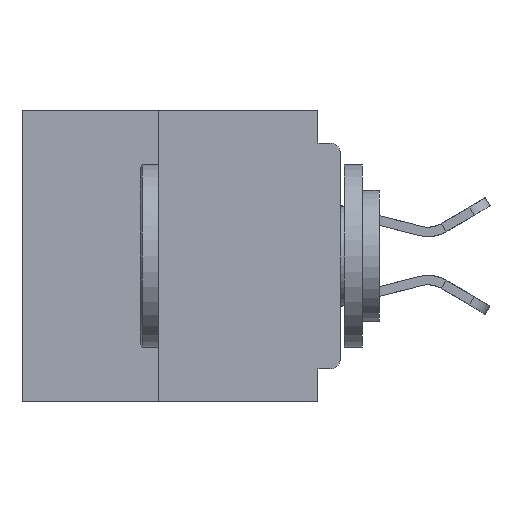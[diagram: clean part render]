
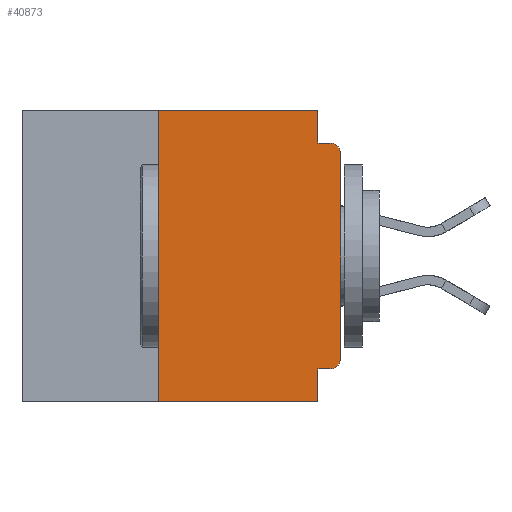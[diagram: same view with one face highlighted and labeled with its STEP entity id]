
A CAD part, left-side view. The second image highlights one B-rep face of the part: STEP entity #40873.
In plain terms, the highlighted planar face has unit normal (-1, 0, 0).
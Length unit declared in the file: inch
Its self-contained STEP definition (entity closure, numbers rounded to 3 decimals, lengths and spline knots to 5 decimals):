
#226 = EDGE_CURVE ( 'NONE', #5020, #37873, #306, .T. ) ;
#306 = CIRCLE ( 'NONE', #12322, 0.015 ) ;
#733 = VECTOR ( 'NONE', #5983, 39.37008 ) ;
#816 = ORIENTED_EDGE ( 'NONE', *, *, #7972, .F. ) ;
#1898 = VERTEX_POINT ( 'NONE', #14434 ) ;
#2320 = DIRECTION ( 'NONE',  ( 0., -1., 0. ) ) ;
#2676 = DIRECTION ( 'NONE',  ( -1., 0., 0. ) ) ;
#4658 = PLANE ( 'NONE',  #10679 ) ;
#4716 = VERTEX_POINT ( 'NONE', #11647 ) ;
#5020 = VERTEX_POINT ( 'NONE', #38479 ) ;
#5144 = LINE ( 'NONE', #42425, #41791 ) ;
#5322 = AXIS2_PLACEMENT_3D ( 'NONE', #24010, #2676, #27599 ) ;
#5771 = CARTESIAN_POINT ( 'NONE',  ( 0., 0.031, 0. ) ) ;
#5791 = VECTOR ( 'NONE', #12923, 39.37008 ) ;
#5983 = DIRECTION ( 'NONE',  ( 0., 0., -1. ) ) ;
#6282 = VECTOR ( 'NONE', #2320, 39.37008 ) ;
#6927 = LINE ( 'NONE', #41256, #5791 ) ;
#7237 = LINE ( 'NONE', #31473, #43775 ) ;
#7409 = LINE ( 'NONE', #44785, #6282 ) ;
#7622 = ORIENTED_EDGE ( 'NONE', *, *, #10558, .F. ) ;
#7972 = EDGE_CURVE ( 'NONE', #29655, #16731, #14196, .T. ) ;
#8274 = DIRECTION ( 'NONE',  ( 0., 0., -1. ) ) ;
#9227 = DIRECTION ( 'NONE',  ( 0., 0., -1. ) ) ;
#9243 = DIRECTION ( 'NONE',  ( -1., 0., 0. ) ) ;
#9346 = CARTESIAN_POINT ( 'NONE',  ( 0., 0.015, -0.06 ) ) ;
#10170 = DIRECTION ( 'NONE',  ( 0., -1., 0. ) ) ;
#10289 = LINE ( 'NONE', #20126, #733 ) ;
#10528 = DIRECTION ( 'NONE',  ( 0., 0., 1. ) ) ;
#10558 = EDGE_CURVE ( 'NONE', #43867, #4716, #6927, .T. ) ;
#10679 = AXIS2_PLACEMENT_3D ( 'NONE', #22403, #29567, #8274 ) ;
#11627 = ORIENTED_EDGE ( 'NONE', *, *, #28068, .F. ) ;
#11647 = CARTESIAN_POINT ( 'NONE',  ( 0., 0.031, -0.045 ) ) ;
#11930 = CARTESIAN_POINT ( 'NONE',  ( 0., 0., -0.355 ) ) ;
#12322 = AXIS2_PLACEMENT_3D ( 'NONE', #9346, #9243, #9227 ) ;
#12923 = DIRECTION ( 'NONE',  ( 0., 0., -1. ) ) ;
#13424 = CARTESIAN_POINT ( 'NONE',  ( 0., 0.031, -0.4 ) ) ;
#14196 = LINE ( 'NONE', #35588, #31994 ) ;
#14434 = CARTESIAN_POINT ( 'NONE',  ( 0., 0.031, -0.355 ) ) ;
#14921 = CARTESIAN_POINT ( 'NONE',  ( 0., 0.015, -0.045 ) ) ;
#15586 = VERTEX_POINT ( 'NONE', #39061 ) ;
#16731 = VERTEX_POINT ( 'NONE', #17220 ) ;
#16990 = CARTESIAN_POINT ( 'NONE',  ( 0., 0.437, -0.4 ) ) ;
#17220 = CARTESIAN_POINT ( 'NONE',  ( 0., 0.25, 0. ) ) ;
#18498 = EDGE_CURVE ( 'NONE', #15586, #5020, #5144, .T. ) ;
#20126 = CARTESIAN_POINT ( 'NONE',  ( 0., 0.031, -0.4 ) ) ;
#21495 = VECTOR ( 'NONE', #29622, 39.37008 ) ;
#21971 = LINE ( 'NONE', #16990, #40803 ) ;
#22266 = FACE_OUTER_BOUND ( 'NONE', #42823, .T. ) ;
#22403 = CARTESIAN_POINT ( 'NONE',  ( 0., 0.437, 0. ) ) ;
#22785 = ORIENTED_EDGE ( 'NONE', *, *, #43940, .T. ) ;
#24010 = CARTESIAN_POINT ( 'NONE',  ( 0., 0.015, -0.34 ) ) ;
#24263 = EDGE_CURVE ( 'NONE', #30639, #15586, #39537, .T. ) ;
#24677 = ORIENTED_EDGE ( 'NONE', *, *, #38551, .F. ) ;
#25369 = ORIENTED_EDGE ( 'NONE', *, *, #33156, .F. ) ;
#27599 = DIRECTION ( 'NONE',  ( 0., 0., -1. ) ) ;
#28068 = EDGE_CURVE ( 'NONE', #30639, #1898, #32102, .T. ) ;
#28243 = CARTESIAN_POINT ( 'NONE',  ( 0., 0.25, -0.4 ) ) ;
#28640 = ORIENTED_EDGE ( 'NONE', *, *, #24263, .T. ) ;
#29567 = DIRECTION ( 'NONE',  ( 1., 0., 0. ) ) ;
#29622 = DIRECTION ( 'NONE',  ( 0., 1., 0. ) ) ;
#29655 = VERTEX_POINT ( 'NONE', #28243 ) ;
#30639 = VERTEX_POINT ( 'NONE', #42014 ) ;
#31473 = CARTESIAN_POINT ( 'NONE',  ( 0., 0.437, 0. ) ) ;
#31734 = ORIENTED_EDGE ( 'NONE', *, *, #18498, .T. ) ;
#31817 = EDGE_CURVE ( 'NONE', #16731, #43867, #7237, .T. ) ;
#31994 = VECTOR ( 'NONE', #10528, 39.37008 ) ;
#32102 = LINE ( 'NONE', #11930, #21495 ) ;
#33156 = EDGE_CURVE ( 'NONE', #4716, #37873, #7409, .T. ) ;
#35588 = CARTESIAN_POINT ( 'NONE',  ( 0., 0.25, -0.4 ) ) ;
#37080 = VERTEX_POINT ( 'NONE', #13424 ) ;
#37873 = VERTEX_POINT ( 'NONE', #14921 ) ;
#38479 = CARTESIAN_POINT ( 'NONE',  ( 0., 0., -0.06 ) ) ;
#38551 = EDGE_CURVE ( 'NONE', #1898, #37080, #10289, .T. ) ;
#39061 = CARTESIAN_POINT ( 'NONE',  ( 0., 0., -0.34 ) ) ;
#39105 = DIRECTION ( 'NONE',  ( 0., 0., 1. ) ) ;
#39537 = CIRCLE ( 'NONE', #5322, 0.015 ) ;
#40192 = ORIENTED_EDGE ( 'NONE', *, *, #226, .T. ) ;
#40803 = VECTOR ( 'NONE', #41756, 39.37008 ) ;
#40873 = ADVANCED_FACE ( 'NONE', ( #22266 ), #4658, .F. ) ;
#41256 = CARTESIAN_POINT ( 'NONE',  ( 0., 0.031, 0. ) ) ;
#41756 = DIRECTION ( 'NONE',  ( 0., -1., 0. ) ) ;
#41791 = VECTOR ( 'NONE', #39105, 39.37008 ) ;
#42014 = CARTESIAN_POINT ( 'NONE',  ( 0., 0.015, -0.355 ) ) ;
#42425 = CARTESIAN_POINT ( 'NONE',  ( 0., 0., 0. ) ) ;
#42823 = EDGE_LOOP ( 'NONE', ( #31734, #40192, #25369, #7622, #43916, #816, #22785, #24677, #11627, #28640 ) ) ;
#43775 = VECTOR ( 'NONE', #10170, 39.37008 ) ;
#43867 = VERTEX_POINT ( 'NONE', #5771 ) ;
#43916 = ORIENTED_EDGE ( 'NONE', *, *, #31817, .F. ) ;
#43940 = EDGE_CURVE ( 'NONE', #29655, #37080, #21971, .T. ) ;
#44785 = CARTESIAN_POINT ( 'NONE',  ( 0., 0., -0.045 ) ) ;
